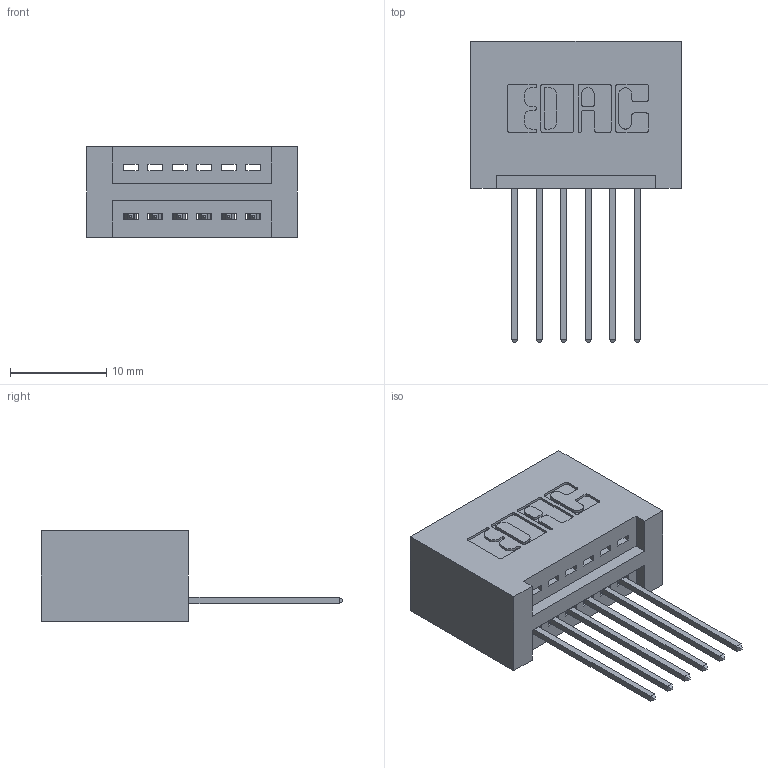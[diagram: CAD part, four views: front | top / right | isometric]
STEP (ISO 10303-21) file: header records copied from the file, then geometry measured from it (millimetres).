
FILE_DESCRIPTION (( 'STEP AP203' ), '1' );
FILE_NAME ('345-006-542-101.STEP', '2018-08-17T00:04:54', ( '' ), ( '' ), 'SwSTEP 2.0', 'SolidWorks 2016', '' );
FILE_SCHEMA (( 'CONFIG_CONTROL_DESIGN' ));
Length unit declared in the file: inch
Products named in the file (3): 345 Part_No Mounting Lugs; 345-292-001_345-293-142; 345-006-542-101
Assembly tree (7 placements, depth 2):
  345-006-542-101
    345 Part_No Mounting Lugs
    345-292-001_345-293-142  x6
Bounding box: 21.84 x 31.29 x 9.4 mm (x, y, z)
Volume: 2377.6 mm3; surface area: 2944.9 mm2
Topology: 7 solids, 7 shells, 466 faces, 1373 edges, 906 vertices
Faces by surface type: plane 316, cylinder 150
Entity records: 9103 total; most frequent: CARTESIAN_POINT 1586, ORIENTED_EDGE 1526, DIRECTION 1431, EDGE_CURVE 763, LINE 615, VECTOR 615, VERTEX_POINT 506, AXIS2_PLACEMENT_3D 408
